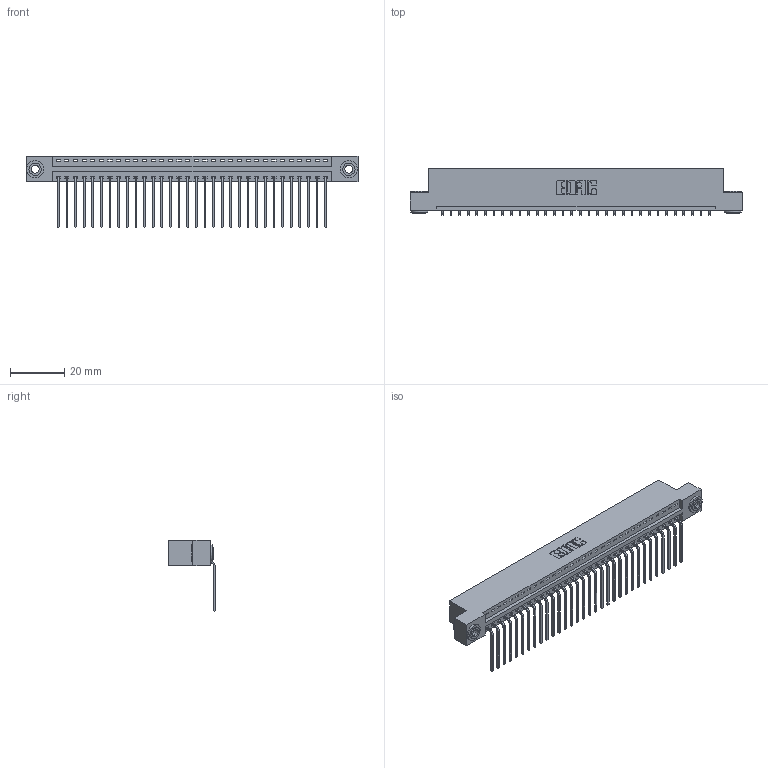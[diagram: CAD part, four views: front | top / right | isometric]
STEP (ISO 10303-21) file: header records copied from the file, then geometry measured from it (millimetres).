
FILE_DESCRIPTION (( 'STEP AP203' ), '1' );
FILE_NAME ('396-032-559-103.STEP', '2019-10-31T21:58:28', ( '' ), ( '' ), 'SwSTEP 2.0', 'SolidWorks 2016', '' );
FILE_SCHEMA (( 'CONFIG_CONTROL_DESIGN' ));
Length unit declared in the file: inch
Products named in the file (4): 345-250-002_345-250-002-102; 396-032-559-103; 346 Part_Flush Mounting Lugs - 0.156 Dia-TH; 345-292-001_558 559 Tail - 1
Assembly tree (35 placements, depth 2):
  396-032-559-103
    346 Part_Flush Mounting Lugs - 0.156 Dia-TH
    345-292-001_558 559 Tail - 1  x32
    345-250-002_345-250-002-102  x2
Bounding box: 122.17 x 17.08 x 26.16 mm (x, y, z)
Volume: 11751.9 mm3; surface area: 15435.6 mm2
Topology: 35 solids, 35 shells, 2080 faces, 6229 edges, 4106 vertices
Faces by surface type: plane 1430, cylinder 642, cone 8
Entity records: 21940 total; most frequent: CARTESIAN_POINT 3743, ORIENTED_EDGE 3702, DIRECTION 3345, EDGE_CURVE 1851, VECTOR 1567, LINE 1567, VERTEX_POINT 1230, AXIS2_PLACEMENT_3D 889
